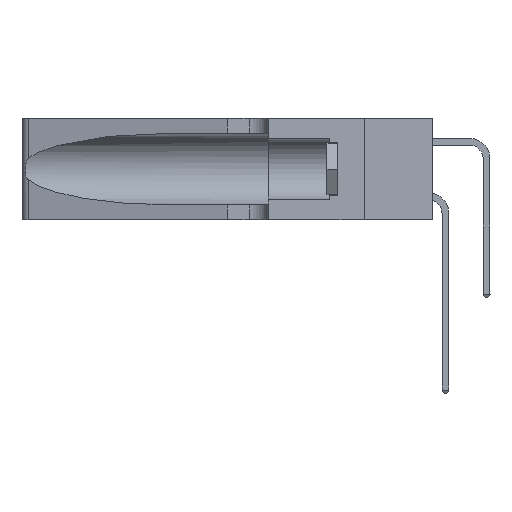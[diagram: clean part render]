
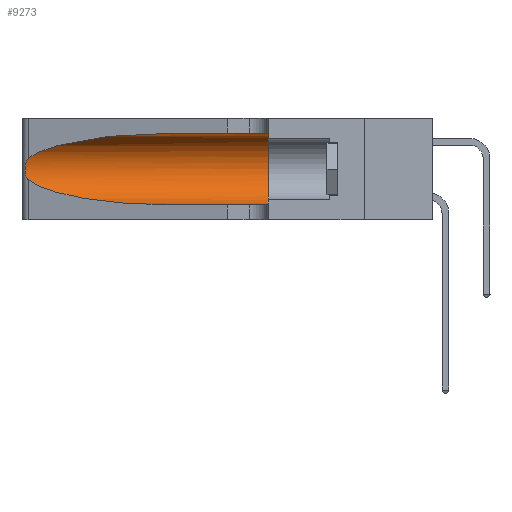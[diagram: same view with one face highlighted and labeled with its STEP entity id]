
A CAD part, left-side view. The second image highlights one B-rep face of the part: STEP entity #9273.
In plain terms, the highlighted cylindrical face has radius 3.308 mm (diameter 6.617 mm), a partial arc.
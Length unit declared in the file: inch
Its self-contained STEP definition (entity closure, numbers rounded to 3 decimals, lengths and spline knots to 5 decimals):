
#692 = CARTESIAN_POINT ( 'NONE',  ( 0.25487, 1.22718, 0.14631 ) ) ;
#833 = CARTESIAN_POINT ( 'NONE',  ( 0.26017, 1.23833, 0.17102 ) ) ;
#1696 = CARTESIAN_POINT ( 'NONE',  ( 0.1305, 0.35, 0.185 ) ) ;
#2542 = VERTEX_POINT ( 'NONE', #29479 ) ;
#5986 = ORIENTED_EDGE ( 'NONE', *, *, #10320, .T. ) ;
#6031 = EDGE_CURVE ( 'NONE', #10942, #2542, #23211, .T. ) ;
#6562 = ORIENTED_EDGE ( 'NONE', *, *, #23061, .F. ) ;
#7237 = CARTESIAN_POINT ( 'NONE',  ( 0.1305, 0.72297, 0.31525 ) ) ;
#7272 = CARTESIAN_POINT ( 'NONE',  ( 0.26018, 1.23835, 0.19895 ) ) ;
#9238 = CARTESIAN_POINT ( 'NONE',  ( 0.1305, 1.61858, 0.31525 ) ) ;
#9273 = ADVANCED_FACE ( 'NONE', ( #25811 ), #26301, .F. ) ;
#9731 = CARTESIAN_POINT ( 'NONE',  ( 0.1305, 1.61858, 0.185 ) ) ;
#10320 = EDGE_CURVE ( 'NONE', #34118, #10942, #11015, .T. ) ;
#10457 =( BOUNDED_CURVE ( )  B_SPLINE_CURVE ( 3, ( #16813, #40193, #17419, #30389 ),
 .UNSPECIFIED., .F., .F. ) 
 B_SPLINE_CURVE_WITH_KNOTS ( ( 4, 4 ),
 ( 1.5708, 2.84003 ),
 .UNSPECIFIED. ) 
 CURVE ( )  GEOMETRIC_REPRESENTATION_ITEM ( )  RATIONAL_B_SPLINE_CURVE ( ( 1., 0.87, 0.87, 1. ) ) 
 REPRESENTATION_ITEM ( '' )  );
#10849 = ORIENTED_EDGE ( 'NONE', *, *, #23973, .F. ) ;
#10942 = VERTEX_POINT ( 'NONE', #12327 ) ;
#11015 = B_SPLINE_CURVE_WITH_KNOTS ( 'NONE', 3,
 ( #13760, #16666, #30508, #40012, #26619, #7272, #27043, #40160, #833, #36552, #39737, #17078, #16933, #692 ),
 .UNSPECIFIED., .F., .F.,
 ( 4, 2, 2, 2, 2, 2, 4 ),
 ( 0., 0.00027, 0.00053, 0.00107, 0.0016, 0.00187, 0.00214 ),
 .UNSPECIFIED. ) ;
#11674 = CARTESIAN_POINT ( 'NONE',  ( 0.25487, 1.22718, 0.22369 ) ) ;
#12065 = EDGE_LOOP ( 'NONE', ( #15010, #5986, #23021, #19750, #10849, #6562 ) ) ;
#12125 = VECTOR ( 'NONE', #15221, 39.37008 ) ;
#12327 = CARTESIAN_POINT ( 'NONE',  ( 0.25487, 1.22718, 0.14631 ) ) ;
#12949 = DIRECTION ( 'NONE',  ( 0., -1., 0. ) ) ;
#13760 = CARTESIAN_POINT ( 'NONE',  ( 0.25487, 1.22718, 0.22369 ) ) ;
#15010 = ORIENTED_EDGE ( 'NONE', *, *, #22150, .T. ) ;
#15221 = DIRECTION ( 'NONE',  ( 0., -1., 0. ) ) ;
#15443 = CARTESIAN_POINT ( 'NONE',  ( 0.1305, 0.35, 0.31525 ) ) ;
#15582 = VERTEX_POINT ( 'NONE', #15443 ) ;
#15953 = CARTESIAN_POINT ( 'NONE',  ( 0.1305, 0.72297, 0.05475 ) ) ;
#16100 = CARTESIAN_POINT ( 'NONE',  ( 0.2373, 1.15595, 0.08982 ) ) ;
#16666 = CARTESIAN_POINT ( 'NONE',  ( 0.25555, 1.22994, 0.2215 ) ) ;
#16813 = CARTESIAN_POINT ( 'NONE',  ( 0.1305, 0.72297, 0.31525 ) ) ;
#16933 = CARTESIAN_POINT ( 'NONE',  ( 0.25555, 1.22993, 0.14849 ) ) ;
#17078 = CARTESIAN_POINT ( 'NONE',  ( 0.25639, 1.23186, 0.15144 ) ) ;
#17419 = CARTESIAN_POINT ( 'NONE',  ( 0.2373, 1.15595, 0.28018 ) ) ;
#18693 = AXIS2_PLACEMENT_3D ( 'NONE', #9731, #19021, #19282 ) ;
#19021 = DIRECTION ( 'NONE',  ( 0., -1., 0. ) ) ;
#19282 = DIRECTION ( 'NONE',  ( 0., 0., -1. ) ) ;
#19298 = AXIS2_PLACEMENT_3D ( 'NONE', #1696, #21575, #30937 ) ;
#19750 = ORIENTED_EDGE ( 'NONE', *, *, #24384, .T. ) ;
#21575 = DIRECTION ( 'NONE',  ( 0., 1., 0. ) ) ;
#21797 = CARTESIAN_POINT ( 'NONE',  ( 0.1305, 0.35, 0.05475 ) ) ;
#22150 = EDGE_CURVE ( 'NONE', #31844, #34118, #10457, .T. ) ;
#22874 = VERTEX_POINT ( 'NONE', #21797 ) ;
#23021 = ORIENTED_EDGE ( 'NONE', *, *, #6031, .T. ) ;
#23061 = EDGE_CURVE ( 'NONE', #31844, #15582, #25667, .T. ) ;
#23211 =( BOUNDED_CURVE ( )  B_SPLINE_CURVE ( 3, ( #42625, #16100, #39430, #15953 ),
 .UNSPECIFIED., .F., .T. ) 
 B_SPLINE_CURVE_WITH_KNOTS ( ( 4, 4 ),
 ( 3.44316, 4.71239 ),
 .UNSPECIFIED. ) 
 CURVE ( )  GEOMETRIC_REPRESENTATION_ITEM ( )  RATIONAL_B_SPLINE_CURVE ( ( 1., 0.87, 0.87, 1. ) ) 
 REPRESENTATION_ITEM ( '' )  );
#23973 = EDGE_CURVE ( 'NONE', #15582, #22874, #33807, .T. ) ;
#24384 = EDGE_CURVE ( 'NONE', #2542, #22874, #37903, .T. ) ;
#24915 = CARTESIAN_POINT ( 'NONE',  ( 0.1305, 1.61858, 0.05475 ) ) ;
#25667 = LINE ( 'NONE', #9238, #31899 ) ;
#25811 = FACE_OUTER_BOUND ( 'NONE', #12065, .T. ) ;
#26301 = CYLINDRICAL_SURFACE ( 'NONE', #18693, 0.13025 ) ;
#26619 = CARTESIAN_POINT ( 'NONE',  ( 0.25854, 1.2359, 0.20912 ) ) ;
#27043 = CARTESIAN_POINT ( 'NONE',  ( 0.26075, 1.23896, 0.19203 ) ) ;
#29479 = CARTESIAN_POINT ( 'NONE',  ( 0.1305, 0.72297, 0.05475 ) ) ;
#30389 = CARTESIAN_POINT ( 'NONE',  ( 0.25487, 1.22718, 0.22369 ) ) ;
#30508 = CARTESIAN_POINT ( 'NONE',  ( 0.25639, 1.23184, 0.21858 ) ) ;
#30937 = DIRECTION ( 'NONE',  ( 0., 0., 1. ) ) ;
#31844 = VERTEX_POINT ( 'NONE', #7237 ) ;
#31899 = VECTOR ( 'NONE', #12949, 39.37008 ) ;
#33807 = CIRCLE ( 'NONE', #19298, 0.13025 ) ;
#34118 = VERTEX_POINT ( 'NONE', #11674 ) ;
#36552 = CARTESIAN_POINT ( 'NONE',  ( 0.25856, 1.23593, 0.16098 ) ) ;
#37903 = LINE ( 'NONE', #24915, #12125 ) ;
#39430 = CARTESIAN_POINT ( 'NONE',  ( 0.18966, 0.96281, 0.05475 ) ) ;
#39737 = CARTESIAN_POINT ( 'NONE',  ( 0.25789, 1.23486, 0.15765 ) ) ;
#40012 = CARTESIAN_POINT ( 'NONE',  ( 0.25787, 1.23484, 0.2124 ) ) ;
#40160 = CARTESIAN_POINT ( 'NONE',  ( 0.26075, 1.23896, 0.178 ) ) ;
#40193 = CARTESIAN_POINT ( 'NONE',  ( 0.18966, 0.96281, 0.31525 ) ) ;
#42625 = CARTESIAN_POINT ( 'NONE',  ( 0.25487, 1.22718, 0.14631 ) ) ;
